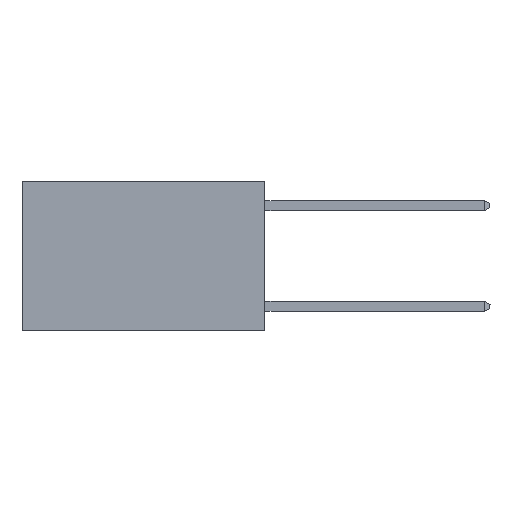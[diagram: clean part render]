
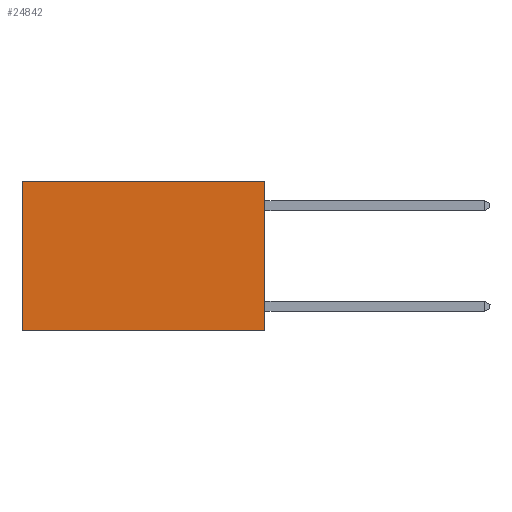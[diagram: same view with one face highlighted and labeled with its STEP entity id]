
A CAD part, left-side view. The second image highlights one B-rep face of the part: STEP entity #24842.
In plain terms, the highlighted planar face has unit normal (-1, 0, 0).
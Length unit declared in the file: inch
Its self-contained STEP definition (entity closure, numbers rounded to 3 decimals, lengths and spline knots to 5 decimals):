
#1438 = PLANE ( 'NONE',  #18230 ) ;
#3306 = ORIENTED_EDGE ( 'NONE', *, *, #16122, .T. ) ;
#3537 = EDGE_CURVE ( 'NONE', #18921, #16155, #27790, .T. ) ;
#3641 = CARTESIAN_POINT ( 'NONE',  ( 0.2625, 0., 0. ) ) ;
#5163 = VECTOR ( 'NONE', #22947, 39.37008 ) ;
#5172 = CARTESIAN_POINT ( 'NONE',  ( 0.2625, 0.6, 0. ) ) ;
#5303 = VECTOR ( 'NONE', #25189, 39.37008 ) ;
#6956 = EDGE_LOOP ( 'NONE', ( #3306, #20932, #12169, #22146 ) ) ;
#7519 = VERTEX_POINT ( 'NONE', #25342 ) ;
#8072 = DIRECTION ( 'NONE',  ( 1., 0., 0. ) ) ;
#8474 = CARTESIAN_POINT ( 'NONE',  ( 0.2625, 0., -0.37 ) ) ;
#10014 = VECTOR ( 'NONE', #12784, 39.37008 ) ;
#10040 = EDGE_CURVE ( 'NONE', #7519, #18921, #27078, .T. ) ;
#10564 = CARTESIAN_POINT ( 'NONE',  ( 0.2625, 0., 0. ) ) ;
#10712 = VECTOR ( 'NONE', #10892, 39.37008 ) ;
#10892 = DIRECTION ( 'NONE',  ( 0., 1., 0. ) ) ;
#11043 = LINE ( 'NONE', #5172, #5163 ) ;
#12169 = ORIENTED_EDGE ( 'NONE', *, *, #10040, .F. ) ;
#12784 = DIRECTION ( 'NONE',  ( 0., 0., -1. ) ) ;
#13125 = CARTESIAN_POINT ( 'NONE',  ( 0.2625, 0., -0.37 ) ) ;
#16122 = EDGE_CURVE ( 'NONE', #26259, #16155, #11043, .T. ) ;
#16155 = VERTEX_POINT ( 'NONE', #25181 ) ;
#18230 = AXIS2_PLACEMENT_3D ( 'NONE', #3641, #8072, #23634 ) ;
#18921 = VERTEX_POINT ( 'NONE', #8474 ) ;
#20932 = ORIENTED_EDGE ( 'NONE', *, *, #3537, .F. ) ;
#21088 = CARTESIAN_POINT ( 'NONE',  ( 0.2625, 0.6, 0. ) ) ;
#22146 = ORIENTED_EDGE ( 'NONE', *, *, #28054, .T. ) ;
#22947 = DIRECTION ( 'NONE',  ( 0., 0., -1. ) ) ;
#22953 = CARTESIAN_POINT ( 'NONE',  ( 0.2625, 0., 0. ) ) ;
#23021 = LINE ( 'NONE', #22953, #5303 ) ;
#23209 = FACE_OUTER_BOUND ( 'NONE', #6956, .T. ) ;
#23634 = DIRECTION ( 'NONE',  ( 0., 0., -1. ) ) ;
#24842 = ADVANCED_FACE ( 'NONE', ( #23209 ), #1438, .F. ) ;
#25181 = CARTESIAN_POINT ( 'NONE',  ( 0.2625, 0.6, -0.37 ) ) ;
#25189 = DIRECTION ( 'NONE',  ( 0., 1., 0. ) ) ;
#25342 = CARTESIAN_POINT ( 'NONE',  ( 0.2625, 0., 0. ) ) ;
#26259 = VERTEX_POINT ( 'NONE', #21088 ) ;
#27078 = LINE ( 'NONE', #10564, #10014 ) ;
#27790 = LINE ( 'NONE', #13125, #10712 ) ;
#28054 = EDGE_CURVE ( 'NONE', #7519, #26259, #23021, .T. ) ;
